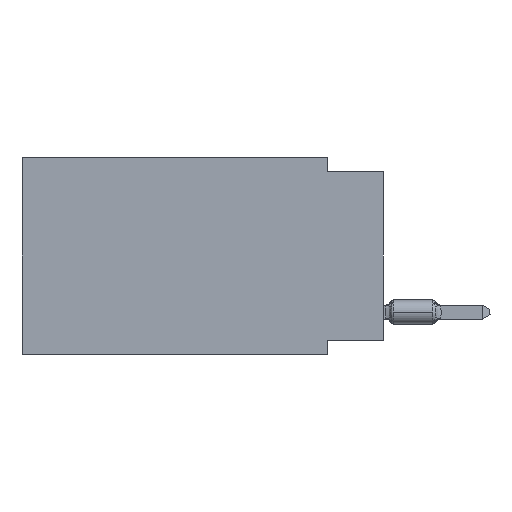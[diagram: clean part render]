
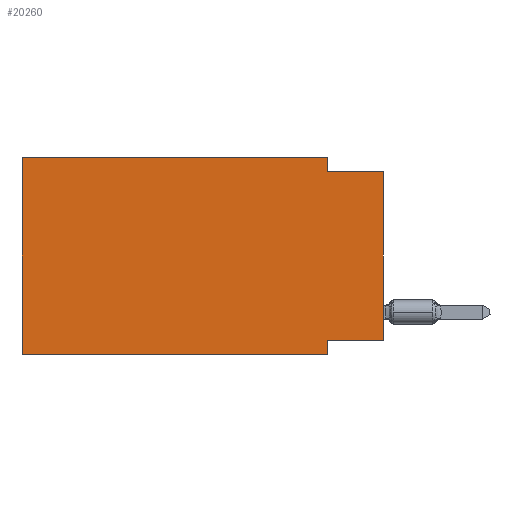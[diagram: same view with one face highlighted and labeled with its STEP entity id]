
A CAD part, left-side view. The second image highlights one B-rep face of the part: STEP entity #20260.
In plain terms, the highlighted planar face has unit normal (-1, 0, 0).
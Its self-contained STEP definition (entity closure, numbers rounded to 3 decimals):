
#2654 = ORIENTED_EDGE ( 'NONE', *, *, #51581, .F. ) ;
#2842 = LINE ( 'NONE', #37973, #71276 ) ;
#5152 = LINE ( 'NONE', #34295, #21422 ) ;
#6242 = DIRECTION ( 'NONE',  ( 0., 0., -1. ) ) ;
#7696 = ORIENTED_EDGE ( 'NONE', *, *, #55331, .F. ) ;
#7953 = CARTESIAN_POINT ( 'NONE',  ( 0., 2.54, 0. ) ) ;
#9118 = CARTESIAN_POINT ( 'NONE',  ( 0., 2.54, -0.635 ) ) ;
#11390 = CARTESIAN_POINT ( 'NONE',  ( 0., 2.54, -8.89 ) ) ;
#12583 = CARTESIAN_POINT ( 'NONE',  ( 0., 0., -8.255 ) ) ;
#13559 = CARTESIAN_POINT ( 'NONE',  ( 0., 0., -0.635 ) ) ;
#13563 = EDGE_CURVE ( 'NONE', #38312, #63078, #18945, .T. ) ;
#14259 = CARTESIAN_POINT ( 'NONE',  ( 0., 16.383, 0. ) ) ;
#14954 = CARTESIAN_POINT ( 'NONE',  ( 0., 2.54, -8.255 ) ) ;
#14972 = EDGE_CURVE ( 'NONE', #63955, #35028, #2842, .T. ) ;
#15937 = ORIENTED_EDGE ( 'NONE', *, *, #58819, .F. ) ;
#17223 = CARTESIAN_POINT ( 'NONE',  ( 0., 0., -8.255 ) ) ;
#17435 = FACE_OUTER_BOUND ( 'NONE', #64955, .T. ) ;
#17806 = PLANE ( 'NONE',  #53969 ) ;
#18066 = VERTEX_POINT ( 'NONE', #7953 ) ;
#18945 = LINE ( 'NONE', #12583, #57992 ) ;
#19165 = VERTEX_POINT ( 'NONE', #42825 ) ;
#19585 = VECTOR ( 'NONE', #31846, 1000. ) ;
#20260 = ADVANCED_FACE ( 'NONE', ( #17435 ), #17806, .F. ) ;
#21422 = VECTOR ( 'NONE', #62312, 1000. ) ;
#24465 = LINE ( 'NONE', #14259, #31019 ) ;
#25512 = LINE ( 'NONE', #60261, #19585 ) ;
#26169 = CARTESIAN_POINT ( 'NONE',  ( 0., 16.383, 0. ) ) ;
#30853 = EDGE_CURVE ( 'NONE', #63078, #55288, #57447, .T. ) ;
#30874 = ORIENTED_EDGE ( 'NONE', *, *, #30853, .F. ) ;
#31019 = VECTOR ( 'NONE', #63689, 1000. ) ;
#31201 = VECTOR ( 'NONE', #32140, 1000. ) ;
#31846 = DIRECTION ( 'NONE',  ( 0., 0., 1. ) ) ;
#32140 = DIRECTION ( 'NONE',  ( 0., 0., 1. ) ) ;
#32509 = LINE ( 'NONE', #26169, #31201 ) ;
#34295 = CARTESIAN_POINT ( 'NONE',  ( 0., 16.383, -8.89 ) ) ;
#35028 = VERTEX_POINT ( 'NONE', #13559 ) ;
#37973 = CARTESIAN_POINT ( 'NONE',  ( 0., 0., -0.635 ) ) ;
#38312 = VERTEX_POINT ( 'NONE', #17223 ) ;
#38391 = LINE ( 'NONE', #69252, #45965 ) ;
#40245 = CARTESIAN_POINT ( 'NONE',  ( 0., 16.383, 0. ) ) ;
#40584 = ORIENTED_EDGE ( 'NONE', *, *, #73563, .T. ) ;
#42825 = CARTESIAN_POINT ( 'NONE',  ( 0., 16.383, 0. ) ) ;
#44296 = ORIENTED_EDGE ( 'NONE', *, *, #14972, .F. ) ;
#45965 = VECTOR ( 'NONE', #72754, 1000. ) ;
#49187 = DIRECTION ( 'NONE',  ( 0., -1., 0. ) ) ;
#49478 = EDGE_CURVE ( 'NONE', #38312, #35028, #25512, .T. ) ;
#51232 = VECTOR ( 'NONE', #68636, 1000. ) ;
#51581 = EDGE_CURVE ( 'NONE', #18066, #63955, #38391, .T. ) ;
#52947 = CARTESIAN_POINT ( 'NONE',  ( 0., 2.54, -8.89 ) ) ;
#53969 = AXIS2_PLACEMENT_3D ( 'NONE', #40245, #63031, #6242 ) ;
#55288 = VERTEX_POINT ( 'NONE', #11390 ) ;
#55331 = EDGE_CURVE ( 'NONE', #19165, #18066, #24465, .T. ) ;
#56846 = VERTEX_POINT ( 'NONE', #61422 ) ;
#56957 = ORIENTED_EDGE ( 'NONE', *, *, #13563, .F. ) ;
#57447 = LINE ( 'NONE', #52947, #51232 ) ;
#57992 = VECTOR ( 'NONE', #69028, 1000. ) ;
#58819 = EDGE_CURVE ( 'NONE', #56846, #19165, #32509, .T. ) ;
#60261 = CARTESIAN_POINT ( 'NONE',  ( 0., 0., 0. ) ) ;
#61422 = CARTESIAN_POINT ( 'NONE',  ( 0., 16.383, -8.89 ) ) ;
#62312 = DIRECTION ( 'NONE',  ( 0., -1., 0. ) ) ;
#63031 = DIRECTION ( 'NONE',  ( 1., 0., 0. ) ) ;
#63078 = VERTEX_POINT ( 'NONE', #14954 ) ;
#63689 = DIRECTION ( 'NONE',  ( 0., -1., 0. ) ) ;
#63955 = VERTEX_POINT ( 'NONE', #9118 ) ;
#64955 = EDGE_LOOP ( 'NONE', ( #65963, #44296, #2654, #7696, #15937, #40584, #30874, #56957 ) ) ;
#65963 = ORIENTED_EDGE ( 'NONE', *, *, #49478, .T. ) ;
#68636 = DIRECTION ( 'NONE',  ( 0., 0., -1. ) ) ;
#69028 = DIRECTION ( 'NONE',  ( 0., 1., 0. ) ) ;
#69252 = CARTESIAN_POINT ( 'NONE',  ( 0., 2.54, 0. ) ) ;
#71276 = VECTOR ( 'NONE', #49187, 1000. ) ;
#72754 = DIRECTION ( 'NONE',  ( 0., 0., -1. ) ) ;
#73563 = EDGE_CURVE ( 'NONE', #56846, #55288, #5152, .T. ) ;
